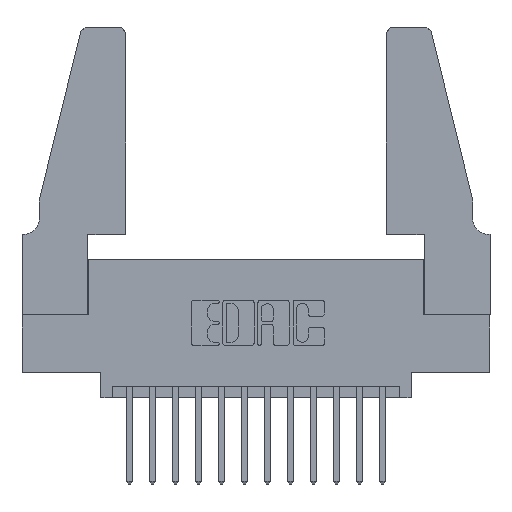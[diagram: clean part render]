
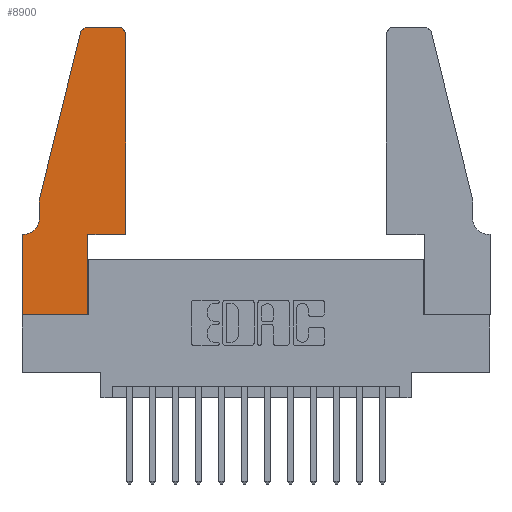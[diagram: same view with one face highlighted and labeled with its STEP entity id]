
A CAD part, top view. The second image highlights one B-rep face of the part: STEP entity #8900.
In plain terms, the highlighted planar face has unit normal (0, 0, 1).
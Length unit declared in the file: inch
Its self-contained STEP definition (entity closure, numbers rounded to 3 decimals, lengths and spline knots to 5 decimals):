
#101 = CARTESIAN_POINT ( 'NONE',  ( 0.0755, 0.42, 0.37 ) ) ;
#188 = VECTOR ( 'NONE', #3863, 39.37008 ) ;
#221 = FACE_OUTER_BOUND ( 'NONE', #8930, .T. ) ;
#315 = VERTEX_POINT ( 'NONE', #8659 ) ;
#563 = VERTEX_POINT ( 'NONE', #14302 ) ;
#600 = CARTESIAN_POINT ( 'NONE',  ( 0.0755, 0.35, 0.37 ) ) ;
#1022 = PLANE ( 'NONE',  #14567 ) ;
#1368 = DIRECTION ( 'NONE',  ( 0., 1., 0. ) ) ;
#1435 = CARTESIAN_POINT ( 'NONE',  ( 0.0755, 0.5, 0.37 ) ) ;
#1436 = ORIENTED_EDGE ( 'NONE', *, *, #4159, .T. ) ;
#1455 = DIRECTION ( 'NONE',  ( 0., 0., -1. ) ) ;
#1520 = DIRECTION ( 'NONE',  ( 0., -1., 0. ) ) ;
#1528 = ORIENTED_EDGE ( 'NONE', *, *, #1946, .T. ) ;
#1594 = EDGE_CURVE ( 'NONE', #5138, #6263, #13071, .T. ) ;
#1851 = DIRECTION ( 'NONE',  ( -1., 0., 0. ) ) ;
#1853 = LINE ( 'NONE', #600, #7949 ) ;
#1946 = EDGE_CURVE ( 'NONE', #10924, #5138, #12115, .T. ) ;
#1970 = ORIENTED_EDGE ( 'NONE', *, *, #12781, .T. ) ;
#2474 = VECTOR ( 'NONE', #1368, 39.37008 ) ;
#2616 = ORIENTED_EDGE ( 'NONE', *, *, #10978, .T. ) ;
#2876 = VERTEX_POINT ( 'NONE', #9025 ) ;
#3272 = AXIS2_PLACEMENT_3D ( 'NONE', #11168, #3896, #12375 ) ;
#3333 = EDGE_CURVE ( 'NONE', #2876, #10924, #13612, .T. ) ;
#3470 = LINE ( 'NONE', #7512, #188 ) ;
#3474 = DIRECTION ( 'NONE',  ( 0., 0., 1. ) ) ;
#3770 = DIRECTION ( 'NONE',  ( 1., 0., 0. ) ) ;
#3863 = DIRECTION ( 'NONE',  ( 0., 1., 0. ) ) ;
#3896 = DIRECTION ( 'NONE',  ( 0., 0., 1. ) ) ;
#3945 = LINE ( 'NONE', #8372, #6831 ) ;
#4159 = EDGE_CURVE ( 'NONE', #15133, #6613, #9085, .T. ) ;
#4726 = CARTESIAN_POINT ( 'NONE',  ( 0.2865, 0., 0.37 ) ) ;
#4761 = CARTESIAN_POINT ( 'NONE',  ( 0.2865, 0.35, 0.37 ) ) ;
#5018 = CARTESIAN_POINT ( 'NONE',  ( 0.0755, 0.5, 0.37 ) ) ;
#5138 = VERTEX_POINT ( 'NONE', #12136 ) ;
#5399 = EDGE_CURVE ( 'NONE', #563, #5553, #11273, .T. ) ;
#5553 = VERTEX_POINT ( 'NONE', #12636 ) ;
#5757 = VERTEX_POINT ( 'NONE', #14287 ) ;
#5856 = VECTOR ( 'NONE', #7763, 39.37008 ) ;
#5952 = CARTESIAN_POINT ( 'NONE',  ( 0.4205, 1.25, 0.37 ) ) ;
#6263 = VERTEX_POINT ( 'NONE', #15226 ) ;
#6283 = DIRECTION ( 'NONE',  ( -0.239, -0.971, 0. ) ) ;
#6387 = ORIENTED_EDGE ( 'NONE', *, *, #1594, .T. ) ;
#6613 = VERTEX_POINT ( 'NONE', #101 ) ;
#6650 = EDGE_CURVE ( 'NONE', #6263, #315, #3470, .T. ) ;
#6695 = DIRECTION ( 'NONE',  ( 0., 0., 1. ) ) ;
#6831 = VECTOR ( 'NONE', #15653, 39.37008 ) ;
#7360 = EDGE_CURVE ( 'NONE', #315, #14040, #15111, .T. ) ;
#7373 = EDGE_CURVE ( 'NONE', #5757, #7807, #1853, .T. ) ;
#7446 = LINE ( 'NONE', #5018, #13468 ) ;
#7482 = CARTESIAN_POINT ( 'NONE',  ( 0., 0.35, 0.37 ) ) ;
#7512 = CARTESIAN_POINT ( 'NONE',  ( 0.4505, 0.35, 0.37 ) ) ;
#7546 = VECTOR ( 'NONE', #1520, 39.37008 ) ;
#7638 = CARTESIAN_POINT ( 'NONE',  ( 0., 0., 0.37 ) ) ;
#7763 = DIRECTION ( 'NONE',  ( 0., -1., 0. ) ) ;
#7807 = VERTEX_POINT ( 'NONE', #7482 ) ;
#7897 = EDGE_CURVE ( 'NONE', #7807, #2876, #7937, .T. ) ;
#7937 = LINE ( 'NONE', #7638, #7546 ) ;
#7949 = VECTOR ( 'NONE', #1851, 39.37008 ) ;
#8372 = CARTESIAN_POINT ( 'NONE',  ( 0.2605, 1.25, 0.37 ) ) ;
#8659 = CARTESIAN_POINT ( 'NONE',  ( 0.4505, 1.22, 0.37 ) ) ;
#8755 = CARTESIAN_POINT ( 'NONE',  ( 0.0055, 0.42, 0.37 ) ) ;
#8900 = ADVANCED_FACE ( 'NONE', ( #221 ), #1022, .T. ) ;
#8930 = EDGE_LOOP ( 'NONE', ( #1970, #9034, #10979, #1436, #2616, #11870, #15786, #12701, #1528, #6387, #14793, #10680 ) ) ;
#9025 = CARTESIAN_POINT ( 'NONE',  ( 0., 0., 0.37 ) ) ;
#9034 = ORIENTED_EDGE ( 'NONE', *, *, #5399, .T. ) ;
#9085 = LINE ( 'NONE', #13759, #5856 ) ;
#9551 = CARTESIAN_POINT ( 'NONE',  ( 0., 0.35, 0.37 ) ) ;
#9841 = CARTESIAN_POINT ( 'NONE',  ( 0., 0., 0.37 ) ) ;
#9887 = VECTOR ( 'NONE', #12698, 39.37008 ) ;
#9952 = DIRECTION ( 'NONE',  ( -1., 0., 0. ) ) ;
#10260 = CIRCLE ( 'NONE', #14190, 0.07 ) ;
#10406 = VECTOR ( 'NONE', #3770, 39.37008 ) ;
#10680 = ORIENTED_EDGE ( 'NONE', *, *, #7360, .T. ) ;
#10924 = VERTEX_POINT ( 'NONE', #4726 ) ;
#10978 = EDGE_CURVE ( 'NONE', #6613, #5757, #10260, .T. ) ;
#10979 = ORIENTED_EDGE ( 'NONE', *, *, #11597, .T. ) ;
#11168 = CARTESIAN_POINT ( 'NONE',  ( 0.284, 1.22, 0.37 ) ) ;
#11273 = CIRCLE ( 'NONE', #3272, 0.03 ) ;
#11597 = EDGE_CURVE ( 'NONE', #5553, #15133, #7446, .T. ) ;
#11870 = ORIENTED_EDGE ( 'NONE', *, *, #7373, .T. ) ;
#11934 = DIRECTION ( 'NONE',  ( 1., 0., 0. ) ) ;
#12003 = AXIS2_PLACEMENT_3D ( 'NONE', #13918, #6695, #15141 ) ;
#12115 = LINE ( 'NONE', #4761, #2474 ) ;
#12136 = CARTESIAN_POINT ( 'NONE',  ( 0.2865, 0.35, 0.37 ) ) ;
#12375 = DIRECTION ( 'NONE',  ( 1., 0., 0. ) ) ;
#12636 = CARTESIAN_POINT ( 'NONE',  ( 0.25487, 1.22718, 0.37 ) ) ;
#12698 = DIRECTION ( 'NONE',  ( 1., 0., 0. ) ) ;
#12701 = ORIENTED_EDGE ( 'NONE', *, *, #3333, .T. ) ;
#12781 = EDGE_CURVE ( 'NONE', #14040, #563, #3945, .T. ) ;
#13071 = LINE ( 'NONE', #14469, #9887 ) ;
#13468 = VECTOR ( 'NONE', #6283, 39.37008 ) ;
#13612 = LINE ( 'NONE', #9841, #10406 ) ;
#13759 = CARTESIAN_POINT ( 'NONE',  ( 0.0755, 0.5, 0.37 ) ) ;
#13918 = CARTESIAN_POINT ( 'NONE',  ( 0.4205, 1.22, 0.37 ) ) ;
#14040 = VERTEX_POINT ( 'NONE', #5952 ) ;
#14190 = AXIS2_PLACEMENT_3D ( 'NONE', #8755, #1455, #9952 ) ;
#14287 = CARTESIAN_POINT ( 'NONE',  ( 0.0055, 0.35, 0.37 ) ) ;
#14302 = CARTESIAN_POINT ( 'NONE',  ( 0.284, 1.25, 0.37 ) ) ;
#14469 = CARTESIAN_POINT ( 'NONE',  ( 0.4505, 0.35, 0.37 ) ) ;
#14567 = AXIS2_PLACEMENT_3D ( 'NONE', #9551, #3474, #11934 ) ;
#14793 = ORIENTED_EDGE ( 'NONE', *, *, #6650, .T. ) ;
#15111 = CIRCLE ( 'NONE', #12003, 0.03 ) ;
#15133 = VERTEX_POINT ( 'NONE', #1435 ) ;
#15141 = DIRECTION ( 'NONE',  ( 1., 0., 0. ) ) ;
#15226 = CARTESIAN_POINT ( 'NONE',  ( 0.4505, 0.35, 0.37 ) ) ;
#15653 = DIRECTION ( 'NONE',  ( -1., 0., 0. ) ) ;
#15786 = ORIENTED_EDGE ( 'NONE', *, *, #7897, .T. ) ;
